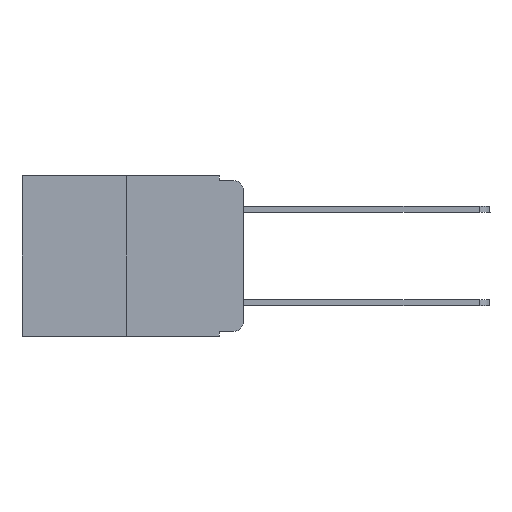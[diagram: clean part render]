
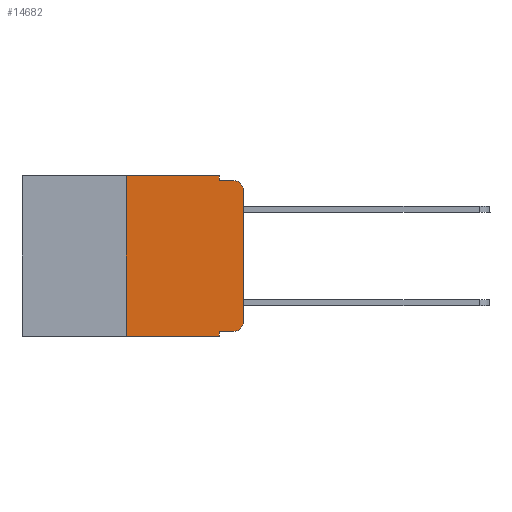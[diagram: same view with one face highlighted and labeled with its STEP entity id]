
A CAD part, left-side view. The second image highlights one B-rep face of the part: STEP entity #14682.
In plain terms, the highlighted planar face has unit normal (-1, 0, 0).
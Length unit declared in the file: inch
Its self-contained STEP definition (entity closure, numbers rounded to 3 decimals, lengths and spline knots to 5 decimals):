
#273 = VECTOR ( 'NONE', #9603, 39.37008 ) ;
#297 = DIRECTION ( 'NONE',  ( -1., 0., 0. ) ) ;
#465 = EDGE_CURVE ( 'NONE', #962, #18603, #16983, .T. ) ;
#875 = VECTOR ( 'NONE', #16060, 39.37008 ) ;
#962 = VERTEX_POINT ( 'NONE', #6994 ) ;
#1107 = ORIENTED_EDGE ( 'NONE', *, *, #1203, .T. ) ;
#1203 = EDGE_CURVE ( 'NONE', #5561, #22912, #2288, .T. ) ;
#1873 = DIRECTION ( 'NONE',  ( 1., 0., 0. ) ) ;
#1985 = DIRECTION ( 'NONE',  ( 0., 0., 1. ) ) ;
#2288 = CIRCLE ( 'NONE', #8860, 0.02 ) ;
#2338 = VECTOR ( 'NONE', #1985, 39.37008 ) ;
#2502 = EDGE_CURVE ( 'NONE', #16512, #17198, #7878, .T. ) ;
#3577 = DIRECTION ( 'NONE',  ( 0., 0., -1. ) ) ;
#3642 = CARTESIAN_POINT ( 'NONE',  ( 0., 0.02, -0.333 ) ) ;
#4477 = EDGE_LOOP ( 'NONE', ( #9065, #1107, #21056, #10546, #9444, #16801, #13569, #18803, #19655, #14906 ) ) ;
#4711 = CARTESIAN_POINT ( 'NONE',  ( 0., 0.051, -0.333 ) ) ;
#5346 = DIRECTION ( 'NONE',  ( 0., 0., -1. ) ) ;
#5363 = EDGE_CURVE ( 'NONE', #13331, #962, #12441, .T. ) ;
#5561 = VERTEX_POINT ( 'NONE', #7649 ) ;
#6109 = LINE ( 'NONE', #14374, #875 ) ;
#6424 = EDGE_CURVE ( 'NONE', #16512, #22723, #24883, .T. ) ;
#6994 = CARTESIAN_POINT ( 'NONE',  ( 0., 0.25, 0. ) ) ;
#7072 = EDGE_CURVE ( 'NONE', #17198, #16548, #11660, .T. ) ;
#7649 = CARTESIAN_POINT ( 'NONE',  ( 0., 0., -0.03 ) ) ;
#7765 = CARTESIAN_POINT ( 'NONE',  ( 0., 0., 0. ) ) ;
#7878 = LINE ( 'NONE', #21726, #17025 ) ;
#8397 = CARTESIAN_POINT ( 'NONE',  ( 0., 0.02, -0.03 ) ) ;
#8828 = CARTESIAN_POINT ( 'NONE',  ( 0., 0.473, 0. ) ) ;
#8860 = AXIS2_PLACEMENT_3D ( 'NONE', #8397, #297, #9944 ) ;
#9065 = ORIENTED_EDGE ( 'NONE', *, *, #16814, .T. ) ;
#9444 = ORIENTED_EDGE ( 'NONE', *, *, #465, .F. ) ;
#9603 = DIRECTION ( 'NONE',  ( 0., -1., 0. ) ) ;
#9841 = CARTESIAN_POINT ( 'NONE',  ( 0., 0.051, 0. ) ) ;
#9941 = CARTESIAN_POINT ( 'NONE',  ( 0., 0.02, -0.01 ) ) ;
#9944 = DIRECTION ( 'NONE',  ( 0., 0., -1. ) ) ;
#10389 = CARTESIAN_POINT ( 'NONE',  ( 0., 0., -0.313 ) ) ;
#10546 = ORIENTED_EDGE ( 'NONE', *, *, #14779, .F. ) ;
#10778 = DIRECTION ( 'NONE',  ( 0., -1., 0. ) ) ;
#10858 = CARTESIAN_POINT ( 'NONE',  ( 0., 0.051, 0. ) ) ;
#11065 = CARTESIAN_POINT ( 'NONE',  ( 0., 0.051, 0. ) ) ;
#11428 = FACE_OUTER_BOUND ( 'NONE', #4477, .T. ) ;
#11660 = CIRCLE ( 'NONE', #23630, 0.02 ) ;
#11673 = LINE ( 'NONE', #23305, #273 ) ;
#12065 = VECTOR ( 'NONE', #3577, 39.37008 ) ;
#12292 = DIRECTION ( 'NONE',  ( -1., 0., 0. ) ) ;
#12441 = LINE ( 'NONE', #14012, #18058 ) ;
#13188 = CARTESIAN_POINT ( 'NONE',  ( 0., 0.051, -0.343 ) ) ;
#13225 = CARTESIAN_POINT ( 'NONE',  ( 0., 0.473, 0. ) ) ;
#13331 = VERTEX_POINT ( 'NONE', #25455 ) ;
#13569 = ORIENTED_EDGE ( 'NONE', *, *, #20024, .T. ) ;
#13999 = DIRECTION ( 'NONE',  ( 0., 0., -1. ) ) ;
#14012 = CARTESIAN_POINT ( 'NONE',  ( 0., 0.25, 0. ) ) ;
#14374 = CARTESIAN_POINT ( 'NONE',  ( 0., 0.473, -0.343 ) ) ;
#14498 = VERTEX_POINT ( 'NONE', #24864 ) ;
#14682 = ADVANCED_FACE ( 'NONE', ( #11428 ), #19562, .F. ) ;
#14779 = EDGE_CURVE ( 'NONE', #18603, #14498, #25486, .T. ) ;
#14906 = ORIENTED_EDGE ( 'NONE', *, *, #7072, .T. ) ;
#14912 = AXIS2_PLACEMENT_3D ( 'NONE', #13225, #1873, #5346 ) ;
#15950 = EDGE_CURVE ( 'NONE', #14498, #22912, #11673, .T. ) ;
#16060 = DIRECTION ( 'NONE',  ( 0., -1., 0. ) ) ;
#16512 = VERTEX_POINT ( 'NONE', #4711 ) ;
#16548 = VERTEX_POINT ( 'NONE', #10389 ) ;
#16801 = ORIENTED_EDGE ( 'NONE', *, *, #5363, .F. ) ;
#16814 = EDGE_CURVE ( 'NONE', #16548, #5561, #21744, .T. ) ;
#16983 = LINE ( 'NONE', #8828, #24973 ) ;
#17025 = VECTOR ( 'NONE', #24727, 39.37008 ) ;
#17198 = VERTEX_POINT ( 'NONE', #3642 ) ;
#18058 = VECTOR ( 'NONE', #21887, 39.37008 ) ;
#18603 = VERTEX_POINT ( 'NONE', #10858 ) ;
#18803 = ORIENTED_EDGE ( 'NONE', *, *, #6424, .F. ) ;
#19562 = PLANE ( 'NONE',  #14912 ) ;
#19655 = ORIENTED_EDGE ( 'NONE', *, *, #2502, .T. ) ;
#20024 = EDGE_CURVE ( 'NONE', #13331, #22723, #6109, .T. ) ;
#20174 = CARTESIAN_POINT ( 'NONE',  ( 0., 0.02, -0.313 ) ) ;
#21056 = ORIENTED_EDGE ( 'NONE', *, *, #15950, .F. ) ;
#21726 = CARTESIAN_POINT ( 'NONE',  ( 0., 0.051, -0.333 ) ) ;
#21744 = LINE ( 'NONE', #7765, #2338 ) ;
#21887 = DIRECTION ( 'NONE',  ( 0., 0., 1. ) ) ;
#22723 = VERTEX_POINT ( 'NONE', #13188 ) ;
#22912 = VERTEX_POINT ( 'NONE', #9941 ) ;
#23305 = CARTESIAN_POINT ( 'NONE',  ( 0., 0.051, -0.01 ) ) ;
#23630 = AXIS2_PLACEMENT_3D ( 'NONE', #20174, #12292, #24289 ) ;
#24289 = DIRECTION ( 'NONE',  ( 0., 0., -1. ) ) ;
#24386 = VECTOR ( 'NONE', #13999, 39.37008 ) ;
#24727 = DIRECTION ( 'NONE',  ( 0., -1., 0. ) ) ;
#24864 = CARTESIAN_POINT ( 'NONE',  ( 0., 0.051, -0.01 ) ) ;
#24883 = LINE ( 'NONE', #11065, #12065 ) ;
#24973 = VECTOR ( 'NONE', #10778, 39.37008 ) ;
#25455 = CARTESIAN_POINT ( 'NONE',  ( 0., 0.25, -0.343 ) ) ;
#25486 = LINE ( 'NONE', #9841, #24386 ) ;
